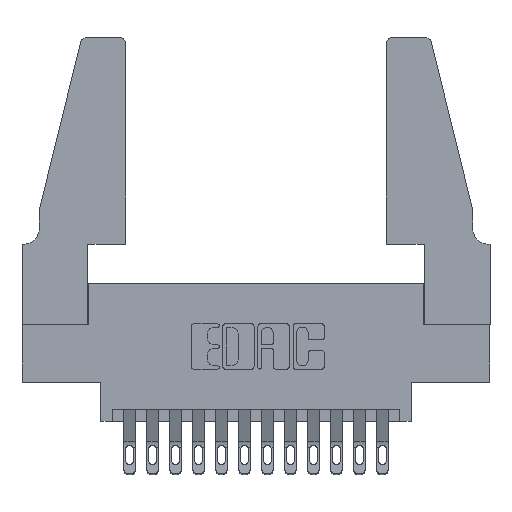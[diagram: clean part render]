
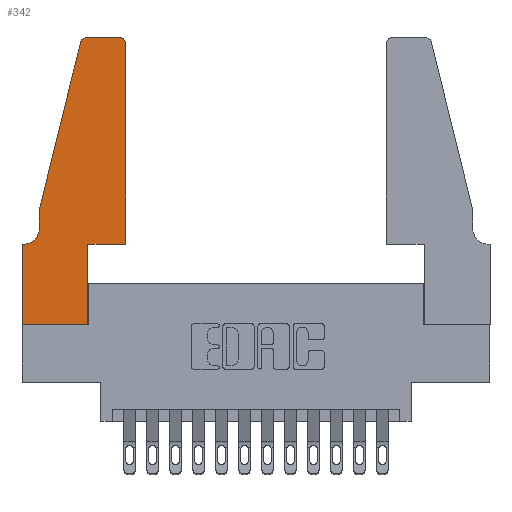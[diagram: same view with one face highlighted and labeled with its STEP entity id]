
A CAD part, top view. The second image highlights one B-rep face of the part: STEP entity #342.
In plain terms, the highlighted planar face has unit normal (0, 0, 1).
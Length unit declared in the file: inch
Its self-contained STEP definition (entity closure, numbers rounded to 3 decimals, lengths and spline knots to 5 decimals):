
#46 = EDGE_LOOP ( 'NONE', ( #7720, #10873, #13753, #15208, #10182, #3492, #4950, #12641, #10276, #11400, #14567, #14697 ) ) ;
#137 = CARTESIAN_POINT ( 'NONE',  ( 0.0755, 0.5, 0.37 ) ) ;
#220 = VERTEX_POINT ( 'NONE', #14535 ) ;
#240 = DIRECTION ( 'NONE',  ( 0., 1., 0. ) ) ;
#342 = ADVANCED_FACE ( 'NONE', ( #5992 ), #4618, .T. ) ;
#746 = LINE ( 'NONE', #12227, #14359 ) ;
#754 = CARTESIAN_POINT ( 'NONE',  ( 0., 0., 0.37 ) ) ;
#806 = LINE ( 'NONE', #15143, #10370 ) ;
#905 = AXIS2_PLACEMENT_3D ( 'NONE', #14732, #8586, #13400 ) ;
#1158 = DIRECTION ( 'NONE',  ( 0., 0., -1. ) ) ;
#1178 = DIRECTION ( 'NONE',  ( -0.239, -0.971, 0. ) ) ;
#1181 = VECTOR ( 'NONE', #14704, 39.37008 ) ;
#1340 = CARTESIAN_POINT ( 'NONE',  ( 0.2865, 0.35, 0.37 ) ) ;
#1617 = EDGE_CURVE ( 'NONE', #9641, #11542, #13321, .T. ) ;
#1809 = EDGE_CURVE ( 'NONE', #7075, #8204, #15260, .T. ) ;
#1946 = CARTESIAN_POINT ( 'NONE',  ( 0.0055, 0.35, 0.37 ) ) ;
#2686 = CARTESIAN_POINT ( 'NONE',  ( 0.4505, 0.35, 0.37 ) ) ;
#3236 = LINE ( 'NONE', #9416, #12770 ) ;
#3492 = ORIENTED_EDGE ( 'NONE', *, *, #6030, .T. ) ;
#4001 = VECTOR ( 'NONE', #240, 39.37008 ) ;
#4022 = CARTESIAN_POINT ( 'NONE',  ( 0., 0., 0.37 ) ) ;
#4618 = PLANE ( 'NONE',  #10759 ) ;
#4796 = CIRCLE ( 'NONE', #12696, 0.03 ) ;
#4950 = ORIENTED_EDGE ( 'NONE', *, *, #1809, .T. ) ;
#4986 = CARTESIAN_POINT ( 'NONE',  ( 0.2865, 0.35, 0.37 ) ) ;
#5847 = VERTEX_POINT ( 'NONE', #8128 ) ;
#5856 = CARTESIAN_POINT ( 'NONE',  ( 0.2605, 1.25, 0.37 ) ) ;
#5913 = DIRECTION ( 'NONE',  ( 1., 0., 0. ) ) ;
#5951 = VECTOR ( 'NONE', #7053, 39.37008 ) ;
#5992 = FACE_OUTER_BOUND ( 'NONE', #46, .T. ) ;
#6012 = CARTESIAN_POINT ( 'NONE',  ( 0.284, 1.22, 0.37 ) ) ;
#6030 = EDGE_CURVE ( 'NONE', #14607, #7075, #806, .T. ) ;
#6228 = VERTEX_POINT ( 'NONE', #9403 ) ;
#6460 = EDGE_CURVE ( 'NONE', #8350, #7749, #7848, .T. ) ;
#7053 = DIRECTION ( 'NONE',  ( 0., -1., 0. ) ) ;
#7075 = VERTEX_POINT ( 'NONE', #15333 ) ;
#7086 = CARTESIAN_POINT ( 'NONE',  ( 0.2865, 0., 0.37 ) ) ;
#7146 = DIRECTION ( 'NONE',  ( 0., 0., 1. ) ) ;
#7661 = EDGE_CURVE ( 'NONE', #8204, #9641, #746, .T. ) ;
#7720 = ORIENTED_EDGE ( 'NONE', *, *, #6460, .T. ) ;
#7749 = VERTEX_POINT ( 'NONE', #10985 ) ;
#7776 = VECTOR ( 'NONE', #1178, 39.37008 ) ;
#7848 = LINE ( 'NONE', #5856, #1181 ) ;
#8128 = CARTESIAN_POINT ( 'NONE',  ( 0.0755, 0.42, 0.37 ) ) ;
#8129 = AXIS2_PLACEMENT_3D ( 'NONE', #13453, #1158, #13516 ) ;
#8204 = VERTEX_POINT ( 'NONE', #4022 ) ;
#8340 = DIRECTION ( 'NONE',  ( -1., 0., 0. ) ) ;
#8350 = VERTEX_POINT ( 'NONE', #11389 ) ;
#8586 = DIRECTION ( 'NONE',  ( 0., 0., 1. ) ) ;
#9180 = EDGE_CURVE ( 'NONE', #6228, #220, #15885, .T. ) ;
#9325 = CARTESIAN_POINT ( 'NONE',  ( 0.4505, 1.22, 0.37 ) ) ;
#9403 = CARTESIAN_POINT ( 'NONE',  ( 0.25487, 1.22718, 0.37 ) ) ;
#9416 = CARTESIAN_POINT ( 'NONE',  ( 0.4505, 0.35, 0.37 ) ) ;
#9559 = EDGE_CURVE ( 'NONE', #220, #5847, #15665, .T. ) ;
#9562 = VERTEX_POINT ( 'NONE', #9325 ) ;
#9641 = VERTEX_POINT ( 'NONE', #7086 ) ;
#9643 = CARTESIAN_POINT ( 'NONE',  ( 0., 0.35, 0.37 ) ) ;
#9734 = EDGE_CURVE ( 'NONE', #5847, #14607, #10271, .T. ) ;
#10069 = DIRECTION ( 'NONE',  ( 0., 1., 0. ) ) ;
#10167 = EDGE_CURVE ( 'NONE', #11542, #13885, #3236, .T. ) ;
#10182 = ORIENTED_EDGE ( 'NONE', *, *, #9734, .T. ) ;
#10229 = LINE ( 'NONE', #13949, #4001 ) ;
#10271 = CIRCLE ( 'NONE', #8129, 0.07 ) ;
#10276 = ORIENTED_EDGE ( 'NONE', *, *, #1617, .T. ) ;
#10320 = EDGE_CURVE ( 'NONE', #7749, #6228, #4796, .T. ) ;
#10370 = VECTOR ( 'NONE', #8340, 39.37008 ) ;
#10396 = CIRCLE ( 'NONE', #905, 0.03 ) ;
#10759 = AXIS2_PLACEMENT_3D ( 'NONE', #9643, #7146, #13451 ) ;
#10873 = ORIENTED_EDGE ( 'NONE', *, *, #10320, .T. ) ;
#10985 = CARTESIAN_POINT ( 'NONE',  ( 0.284, 1.25, 0.37 ) ) ;
#11389 = CARTESIAN_POINT ( 'NONE',  ( 0.4205, 1.25, 0.37 ) ) ;
#11400 = ORIENTED_EDGE ( 'NONE', *, *, #10167, .T. ) ;
#11542 = VERTEX_POINT ( 'NONE', #4986 ) ;
#11712 = DIRECTION ( 'NONE',  ( 1., 0., 0. ) ) ;
#11731 = EDGE_CURVE ( 'NONE', #9562, #8350, #10396, .T. ) ;
#12227 = CARTESIAN_POINT ( 'NONE',  ( 0., 0., 0.37 ) ) ;
#12341 = DIRECTION ( 'NONE',  ( 1., 0., 0. ) ) ;
#12641 = ORIENTED_EDGE ( 'NONE', *, *, #7661, .T. ) ;
#12696 = AXIS2_PLACEMENT_3D ( 'NONE', #6012, #15757, #5913 ) ;
#12770 = VECTOR ( 'NONE', #11712, 39.37008 ) ;
#13038 = CARTESIAN_POINT ( 'NONE',  ( 0.0755, 0.5, 0.37 ) ) ;
#13321 = LINE ( 'NONE', #1340, #13699 ) ;
#13400 = DIRECTION ( 'NONE',  ( 1., 0., 0. ) ) ;
#13451 = DIRECTION ( 'NONE',  ( 1., 0., 0. ) ) ;
#13453 = CARTESIAN_POINT ( 'NONE',  ( 0.0055, 0.42, 0.37 ) ) ;
#13516 = DIRECTION ( 'NONE',  ( -1., 0., 0. ) ) ;
#13699 = VECTOR ( 'NONE', #10069, 39.37008 ) ;
#13726 = VECTOR ( 'NONE', #14274, 39.37008 ) ;
#13753 = ORIENTED_EDGE ( 'NONE', *, *, #9180, .T. ) ;
#13885 = VERTEX_POINT ( 'NONE', #2686 ) ;
#13949 = CARTESIAN_POINT ( 'NONE',  ( 0.4505, 0.35, 0.37 ) ) ;
#14274 = DIRECTION ( 'NONE',  ( 0., -1., 0. ) ) ;
#14359 = VECTOR ( 'NONE', #12341, 39.37008 ) ;
#14535 = CARTESIAN_POINT ( 'NONE',  ( 0.0755, 0.5, 0.37 ) ) ;
#14567 = ORIENTED_EDGE ( 'NONE', *, *, #15537, .T. ) ;
#14607 = VERTEX_POINT ( 'NONE', #1946 ) ;
#14697 = ORIENTED_EDGE ( 'NONE', *, *, #11731, .T. ) ;
#14704 = DIRECTION ( 'NONE',  ( -1., 0., 0. ) ) ;
#14732 = CARTESIAN_POINT ( 'NONE',  ( 0.4205, 1.22, 0.37 ) ) ;
#15143 = CARTESIAN_POINT ( 'NONE',  ( 0.0755, 0.35, 0.37 ) ) ;
#15208 = ORIENTED_EDGE ( 'NONE', *, *, #9559, .T. ) ;
#15260 = LINE ( 'NONE', #754, #5951 ) ;
#15333 = CARTESIAN_POINT ( 'NONE',  ( 0., 0.35, 0.37 ) ) ;
#15537 = EDGE_CURVE ( 'NONE', #13885, #9562, #10229, .T. ) ;
#15665 = LINE ( 'NONE', #13038, #13726 ) ;
#15757 = DIRECTION ( 'NONE',  ( 0., 0., 1. ) ) ;
#15885 = LINE ( 'NONE', #137, #7776 ) ;
